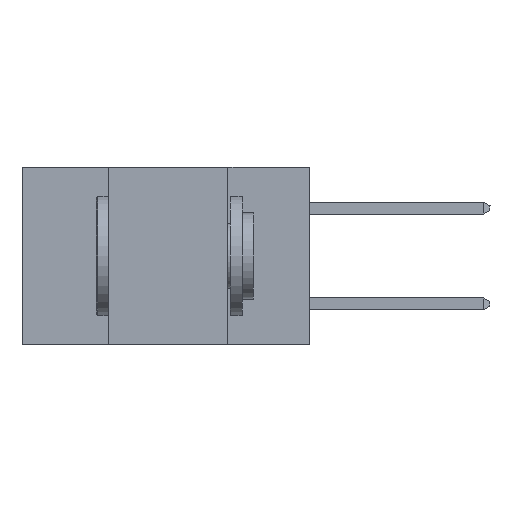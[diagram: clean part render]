
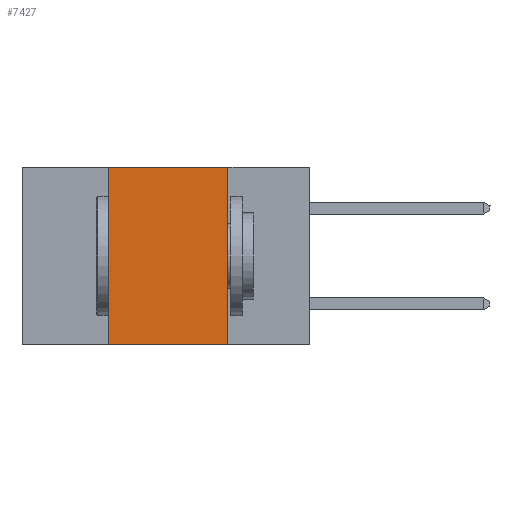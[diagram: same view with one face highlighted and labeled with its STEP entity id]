
A CAD part, left-side view. The second image highlights one B-rep face of the part: STEP entity #7427.
In plain terms, the highlighted planar face has unit normal (-1, 0, 0).
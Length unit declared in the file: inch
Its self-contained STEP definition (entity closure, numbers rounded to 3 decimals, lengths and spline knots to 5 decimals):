
#1373 = EDGE_LOOP ( 'NONE', ( #9839, #23852, #22292, #30175 ) ) ;
#2116 = CARTESIAN_POINT ( 'NONE',  ( 0., 0.42, 0. ) ) ;
#2867 = AXIS2_PLACEMENT_3D ( 'NONE', #17157, #24167, #31058 ) ;
#3324 = FACE_OUTER_BOUND ( 'NONE', #1373, .T. ) ;
#3502 = EDGE_CURVE ( 'NONE', #15321, #10660, #31949, .T. ) ;
#4024 = VECTOR ( 'NONE', #14880, 39.37008 ) ;
#4600 = VERTEX_POINT ( 'NONE', #12396 ) ;
#6579 = VERTEX_POINT ( 'NONE', #2116 ) ;
#6952 = DIRECTION ( 'NONE',  ( 0., 0., -1. ) ) ;
#7427 = ADVANCED_FACE ( 'NONE', ( #3324 ), #30707, .F. ) ;
#9839 = ORIENTED_EDGE ( 'NONE', *, *, #33557, .F. ) ;
#10236 = CARTESIAN_POINT ( 'NONE',  ( 0., 0.42, -0.37 ) ) ;
#10660 = VERTEX_POINT ( 'NONE', #12531 ) ;
#12396 = CARTESIAN_POINT ( 'NONE',  ( 0., 0.17, 0. ) ) ;
#12531 = CARTESIAN_POINT ( 'NONE',  ( 0., 0.17, -0.37 ) ) ;
#14880 = DIRECTION ( 'NONE',  ( 0., 0., 1. ) ) ;
#15321 = VERTEX_POINT ( 'NONE', #10236 ) ;
#17157 = CARTESIAN_POINT ( 'NONE',  ( 0., 0.6, 0. ) ) ;
#17172 = CARTESIAN_POINT ( 'NONE',  ( 0., 0.17, 0. ) ) ;
#19470 = VECTOR ( 'NONE', #29079, 39.37008 ) ;
#21042 = VECTOR ( 'NONE', #6952, 39.37008 ) ;
#21614 = EDGE_CURVE ( 'NONE', #6579, #4600, #34953, .T. ) ;
#22292 = ORIENTED_EDGE ( 'NONE', *, *, #28294, .F. ) ;
#23852 = ORIENTED_EDGE ( 'NONE', *, *, #21614, .F. ) ;
#24167 = DIRECTION ( 'NONE',  ( 1., 0., 0. ) ) ;
#25647 = LINE ( 'NONE', #28932, #4024 ) ;
#26831 = CARTESIAN_POINT ( 'NONE',  ( 0., 0.6, -0.37 ) ) ;
#27691 = VECTOR ( 'NONE', #31630, 39.37008 ) ;
#28264 = CARTESIAN_POINT ( 'NONE',  ( 0., 0.6, 0. ) ) ;
#28294 = EDGE_CURVE ( 'NONE', #15321, #6579, #25647, .T. ) ;
#28932 = CARTESIAN_POINT ( 'NONE',  ( 0., 0.42, 0. ) ) ;
#29079 = DIRECTION ( 'NONE',  ( 0., -1., 0. ) ) ;
#30175 = ORIENTED_EDGE ( 'NONE', *, *, #3502, .T. ) ;
#30707 = PLANE ( 'NONE',  #2867 ) ;
#31058 = DIRECTION ( 'NONE',  ( 0., 0., -1. ) ) ;
#31630 = DIRECTION ( 'NONE',  ( 0., -1., 0. ) ) ;
#31949 = LINE ( 'NONE', #26831, #19470 ) ;
#33557 = EDGE_CURVE ( 'NONE', #4600, #10660, #34243, .T. ) ;
#34243 = LINE ( 'NONE', #17172, #21042 ) ;
#34953 = LINE ( 'NONE', #28264, #27691 ) ;
